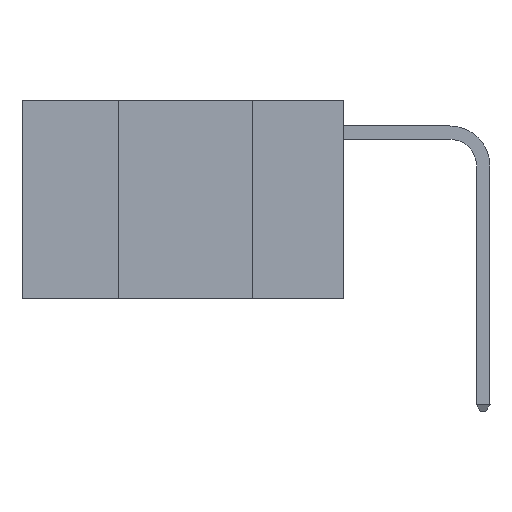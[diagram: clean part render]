
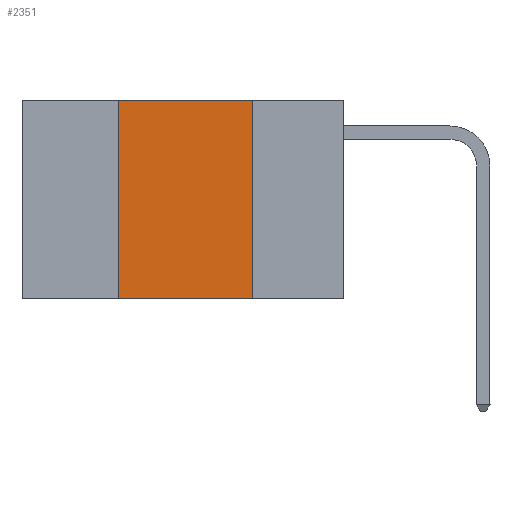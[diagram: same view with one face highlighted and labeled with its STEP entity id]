
A CAD part, left-side view. The second image highlights one B-rep face of the part: STEP entity #2351.
In plain terms, the highlighted planar face has unit normal (-1, 0, 0).
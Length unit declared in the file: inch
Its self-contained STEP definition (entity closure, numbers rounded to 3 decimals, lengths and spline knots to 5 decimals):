
#1956 = VECTOR ( 'NONE', #8914, 39.37008 ) ;
#2161 = FACE_OUTER_BOUND ( 'NONE', #14585, .T. ) ;
#2201 = VECTOR ( 'NONE', #4790, 39.37008 ) ;
#2351 = ADVANCED_FACE ( 'NONE', ( #2161 ), #13217, .F. ) ;
#3225 = CARTESIAN_POINT ( 'NONE',  ( 0., 0.17, 0. ) ) ;
#3537 = ORIENTED_EDGE ( 'NONE', *, *, #15089, .F. ) ;
#3555 = ORIENTED_EDGE ( 'NONE', *, *, #9582, .F. ) ;
#3687 = ORIENTED_EDGE ( 'NONE', *, *, #13595, .F. ) ;
#3699 = ORIENTED_EDGE ( 'NONE', *, *, #12810, .T. ) ;
#4783 = CARTESIAN_POINT ( 'NONE',  ( 0., 0.6, -0.37 ) ) ;
#4790 = DIRECTION ( 'NONE',  ( 0., -1., 0. ) ) ;
#5383 = LINE ( 'NONE', #3225, #14513 ) ;
#5440 = CARTESIAN_POINT ( 'NONE',  ( 0., 0.42, 0. ) ) ;
#6060 = CARTESIAN_POINT ( 'NONE',  ( 0., 0.17, 0. ) ) ;
#6546 = VECTOR ( 'NONE', #12040, 39.37008 ) ;
#6852 = VERTEX_POINT ( 'NONE', #11469 ) ;
#8914 = DIRECTION ( 'NONE',  ( 0., 0., 1. ) ) ;
#9547 = CARTESIAN_POINT ( 'NONE',  ( 0., 0.42, -0.37 ) ) ;
#9582 = EDGE_CURVE ( 'NONE', #13135, #10845, #11689, .T. ) ;
#9807 = LINE ( 'NONE', #4783, #6546 ) ;
#10301 = AXIS2_PLACEMENT_3D ( 'NONE', #14964, #14140, #14158 ) ;
#10845 = VERTEX_POINT ( 'NONE', #6060 ) ;
#11218 = VERTEX_POINT ( 'NONE', #9547 ) ;
#11274 = CARTESIAN_POINT ( 'NONE',  ( 0., 0.42, 0. ) ) ;
#11469 = CARTESIAN_POINT ( 'NONE',  ( 0., 0.17, -0.37 ) ) ;
#11689 = LINE ( 'NONE', #12051, #2201 ) ;
#11836 = DIRECTION ( 'NONE',  ( 0., 0., -1. ) ) ;
#12040 = DIRECTION ( 'NONE',  ( 0., -1., 0. ) ) ;
#12051 = CARTESIAN_POINT ( 'NONE',  ( 0., 0.6, 0. ) ) ;
#12810 = EDGE_CURVE ( 'NONE', #11218, #6852, #9807, .T. ) ;
#13135 = VERTEX_POINT ( 'NONE', #5440 ) ;
#13217 = PLANE ( 'NONE',  #10301 ) ;
#13595 = EDGE_CURVE ( 'NONE', #11218, #13135, #14919, .T. ) ;
#14140 = DIRECTION ( 'NONE',  ( 1., 0., 0. ) ) ;
#14158 = DIRECTION ( 'NONE',  ( 0., 0., -1. ) ) ;
#14513 = VECTOR ( 'NONE', #11836, 39.37008 ) ;
#14585 = EDGE_LOOP ( 'NONE', ( #3537, #3555, #3687, #3699 ) ) ;
#14919 = LINE ( 'NONE', #11274, #1956 ) ;
#14964 = CARTESIAN_POINT ( 'NONE',  ( 0., 0.6, 0. ) ) ;
#15089 = EDGE_CURVE ( 'NONE', #10845, #6852, #5383, .T. ) ;
